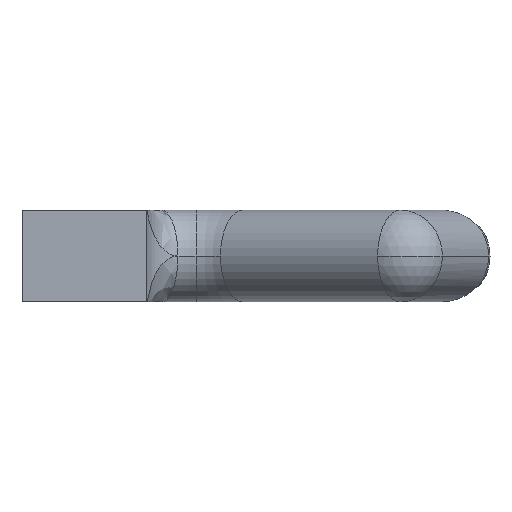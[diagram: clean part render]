
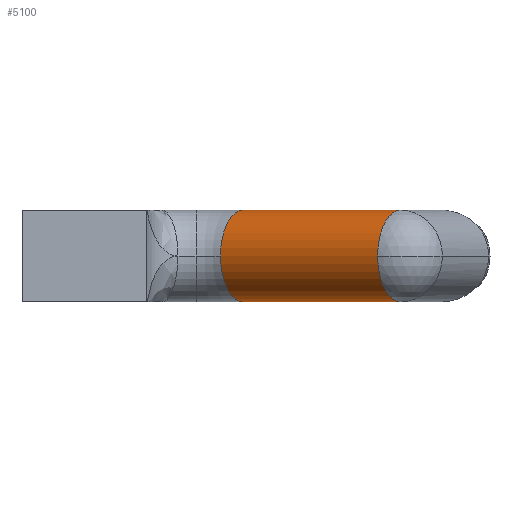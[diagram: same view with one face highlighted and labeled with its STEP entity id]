
A CAD part, left-side view. The second image highlights one B-rep face of the part: STEP entity #5100.
In plain terms, the highlighted cylindrical face has radius 12 mm (diameter 24 mm), a partial arc.
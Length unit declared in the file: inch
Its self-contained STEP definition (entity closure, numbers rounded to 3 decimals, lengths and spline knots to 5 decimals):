
#112 = EDGE_CURVE ( 'NONE', #3696, #5225, #3151, .T. ) ;
#135 = FACE_OUTER_BOUND ( 'NONE', #3212, .T. ) ;
#381 = AXIS2_PLACEMENT_3D ( 'NONE', #5071, #1153, #5728 ) ;
#494 = VECTOR ( 'NONE', #5662, 39.37008 ) ;
#505 = AXIS2_PLACEMENT_3D ( 'NONE', #2234, #6830, #2898 ) ;
#685 = DIRECTION ( 'NONE',  ( -0.491, -0.871, 0. ) ) ;
#992 = CARTESIAN_POINT ( 'NONE',  ( 3.2352, -4.18089, 0. ) ) ;
#997 = EDGE_CURVE ( 'NONE', #2148, #6025, #3523, .T. ) ;
#1045 = CARTESIAN_POINT ( 'NONE',  ( 4.55976, -2.79267, 0.47244 ) ) ;
#1153 = DIRECTION ( 'NONE',  ( 0.491, 0.871, 0. ) ) ;
#1185 = DIRECTION ( 'NONE',  ( 0.871, -0.491, 0. ) ) ;
#1648 = CIRCLE ( 'NONE', #5783, 0.47244 ) ;
#1723 = CARTESIAN_POINT ( 'NONE',  ( 4.20739, -3.41798, 0.47244 ) ) ;
#1724 = CARTESIAN_POINT ( 'NONE',  ( 3.44153, -4.77709, -0.47244 ) ) ;
#1733 = ORIENTED_EDGE ( 'NONE', *, *, #5002, .T. ) ;
#1734 = ORIENTED_EDGE ( 'NONE', *, *, #3317, .T. ) ;
#2075 = CARTESIAN_POINT ( 'NONE',  ( 3.64679, -4.41282, 0.47244 ) ) ;
#2084 = CIRCLE ( 'NONE', #505, 0.47244 ) ;
#2148 = VERTEX_POINT ( 'NONE', #1045 ) ;
#2175 = ORIENTED_EDGE ( 'NONE', *, *, #8101, .F. ) ;
#2234 = CARTESIAN_POINT ( 'NONE',  ( 4.55976, -2.79267, 0. ) ) ;
#2366 = VERTEX_POINT ( 'NONE', #992 ) ;
#2718 = AXIS2_PLACEMENT_3D ( 'NONE', #7744, #3794, #8420 ) ;
#2742 = ORIENTED_EDGE ( 'NONE', *, *, #997, .F. ) ;
#2785 = CARTESIAN_POINT ( 'NONE',  ( 4.55976, -2.79267, -0.47244 ) ) ;
#2898 = DIRECTION ( 'NONE',  ( -0.871, 0.491, 0. ) ) ;
#3151 = LINE ( 'NONE', #1724, #8193 ) ;
#3212 = EDGE_LOOP ( 'NONE', ( #2742, #2175, #4595, #5229, #1733, #1734 ) ) ;
#3317 = EDGE_CURVE ( 'NONE', #2366, #6025, #6717, .T. ) ;
#3460 = CARTESIAN_POINT ( 'NONE',  ( 4.14817, -2.56074, 0. ) ) ;
#3488 = DIRECTION ( 'NONE',  ( 0.491, 0.871, 0. ) ) ;
#3523 = LINE ( 'NONE', #1723, #494 ) ;
#3696 = VERTEX_POINT ( 'NONE', #6782 ) ;
#3794 = DIRECTION ( 'NONE',  ( 0.491, 0.871, 0. ) ) ;
#3808 = CARTESIAN_POINT ( 'NONE',  ( 4.20739, -3.41798, 0. ) ) ;
#4216 = VERTEX_POINT ( 'NONE', #3460 ) ;
#4302 = EDGE_CURVE ( 'NONE', #5225, #4216, #2084, .T. ) ;
#4595 = ORIENTED_EDGE ( 'NONE', *, *, #4302, .F. ) ;
#4997 = DIRECTION ( 'NONE',  ( 0.491, 0.871, 0. ) ) ;
#5002 = EDGE_CURVE ( 'NONE', #3696, #2366, #7318, .T. ) ;
#5071 = CARTESIAN_POINT ( 'NONE',  ( 3.64679, -4.41282, 0. ) ) ;
#5100 = ADVANCED_FACE ( 'NONE', ( #135 ), #5152, .T. ) ;
#5152 = CYLINDRICAL_SURFACE ( 'NONE', #7093, 0.47244 ) ;
#5225 = VERTEX_POINT ( 'NONE', #2785 ) ;
#5229 = ORIENTED_EDGE ( 'NONE', *, *, #112, .F. ) ;
#5662 = DIRECTION ( 'NONE',  ( -0.491, -0.871, 0. ) ) ;
#5728 = DIRECTION ( 'NONE',  ( 0.871, -0.491, 0. ) ) ;
#5783 = AXIS2_PLACEMENT_3D ( 'NONE', #7442, #3488, #8112 ) ;
#6025 = VERTEX_POINT ( 'NONE', #2075 ) ;
#6717 = CIRCLE ( 'NONE', #2718, 0.47244 ) ;
#6782 = CARTESIAN_POINT ( 'NONE',  ( 3.64679, -4.41282, -0.47244 ) ) ;
#6830 = DIRECTION ( 'NONE',  ( 0.491, 0.871, 0. ) ) ;
#7093 = AXIS2_PLACEMENT_3D ( 'NONE', #3808, #685, #1185 ) ;
#7318 = CIRCLE ( 'NONE', #381, 0.47244 ) ;
#7442 = CARTESIAN_POINT ( 'NONE',  ( 4.55976, -2.79267, 0. ) ) ;
#7744 = CARTESIAN_POINT ( 'NONE',  ( 3.64679, -4.41282, 0. ) ) ;
#8101 = EDGE_CURVE ( 'NONE', #4216, #2148, #1648, .T. ) ;
#8112 = DIRECTION ( 'NONE',  ( -0.871, 0.491, 0. ) ) ;
#8193 = VECTOR ( 'NONE', #4997, 39.37008 ) ;
#8420 = DIRECTION ( 'NONE',  ( 0.871, -0.491, 0. ) ) ;
